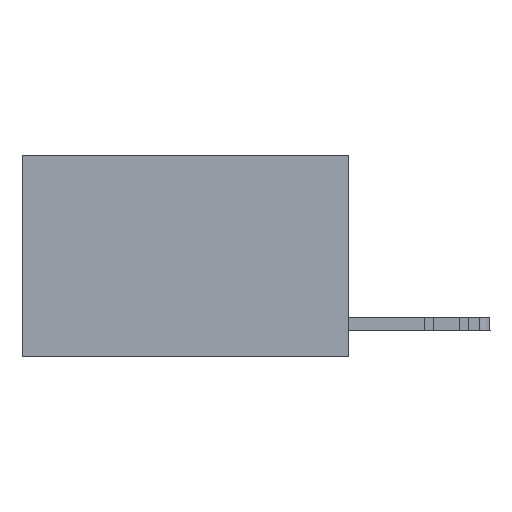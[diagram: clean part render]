
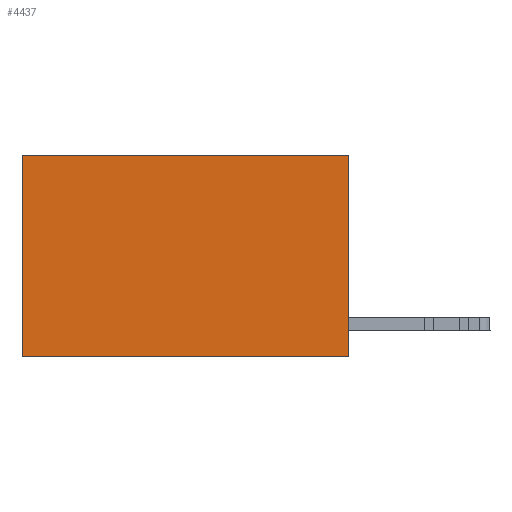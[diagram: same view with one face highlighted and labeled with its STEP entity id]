
A CAD part, left-side view. The second image highlights one B-rep face of the part: STEP entity #4437.
In plain terms, the highlighted planar face has unit normal (-1, 0, 0).
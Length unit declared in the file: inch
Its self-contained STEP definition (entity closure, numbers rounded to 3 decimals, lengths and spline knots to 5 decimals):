
#1441 = LINE ( 'NONE', #10569, #22042 ) ;
#1820 = DIRECTION ( 'NONE',  ( 0., 0., -1. ) ) ;
#1997 = VERTEX_POINT ( 'NONE', #25041 ) ;
#3015 = CARTESIAN_POINT ( 'NONE',  ( 0.2625, 0., -0.37 ) ) ;
#3549 = VERTEX_POINT ( 'NONE', #25917 ) ;
#4223 = LINE ( 'NONE', #25198, #28981 ) ;
#4437 = ADVANCED_FACE ( 'NONE', ( #16709 ), #5034, .F. ) ;
#5034 = PLANE ( 'NONE',  #21243 ) ;
#6851 = CARTESIAN_POINT ( 'NONE',  ( 0.2625, 0., 0. ) ) ;
#7721 = CARTESIAN_POINT ( 'NONE',  ( 0.2625, 0., 0. ) ) ;
#8446 = EDGE_CURVE ( 'NONE', #25374, #1997, #10751, .T. ) ;
#9199 = EDGE_CURVE ( 'NONE', #21931, #25374, #4223, .T. ) ;
#9762 = EDGE_CURVE ( 'NONE', #21931, #3549, #12837, .T. ) ;
#10486 = ORIENTED_EDGE ( 'NONE', *, *, #8446, .F. ) ;
#10569 = CARTESIAN_POINT ( 'NONE',  ( 0.2625, 0.6, 0. ) ) ;
#10751 = LINE ( 'NONE', #13584, #13149 ) ;
#11214 = ORIENTED_EDGE ( 'NONE', *, *, #9199, .F. ) ;
#11903 = DIRECTION ( 'NONE',  ( 0., 0., -1. ) ) ;
#12837 = LINE ( 'NONE', #15709, #16573 ) ;
#13149 = VECTOR ( 'NONE', #17500, 39.37008 ) ;
#13584 = CARTESIAN_POINT ( 'NONE',  ( 0.2625, 0., -0.37 ) ) ;
#15709 = CARTESIAN_POINT ( 'NONE',  ( 0.2625, 0., 0. ) ) ;
#16573 = VECTOR ( 'NONE', #20064, 39.37008 ) ;
#16709 = FACE_OUTER_BOUND ( 'NONE', #27636, .T. ) ;
#17500 = DIRECTION ( 'NONE',  ( 0., 1., 0. ) ) ;
#20064 = DIRECTION ( 'NONE',  ( 0., 1., 0. ) ) ;
#20771 = ORIENTED_EDGE ( 'NONE', *, *, #9762, .T. ) ;
#21243 = AXIS2_PLACEMENT_3D ( 'NONE', #7721, #25990, #11903 ) ;
#21931 = VERTEX_POINT ( 'NONE', #6851 ) ;
#22042 = VECTOR ( 'NONE', #28845, 39.37008 ) ;
#23031 = ORIENTED_EDGE ( 'NONE', *, *, #25968, .T. ) ;
#25041 = CARTESIAN_POINT ( 'NONE',  ( 0.2625, 0.6, -0.37 ) ) ;
#25198 = CARTESIAN_POINT ( 'NONE',  ( 0.2625, 0., 0. ) ) ;
#25374 = VERTEX_POINT ( 'NONE', #3015 ) ;
#25917 = CARTESIAN_POINT ( 'NONE',  ( 0.2625, 0.6, 0. ) ) ;
#25968 = EDGE_CURVE ( 'NONE', #3549, #1997, #1441, .T. ) ;
#25990 = DIRECTION ( 'NONE',  ( 1., 0., 0. ) ) ;
#27636 = EDGE_LOOP ( 'NONE', ( #23031, #10486, #11214, #20771 ) ) ;
#28845 = DIRECTION ( 'NONE',  ( 0., 0., -1. ) ) ;
#28981 = VECTOR ( 'NONE', #1820, 39.37008 ) ;
